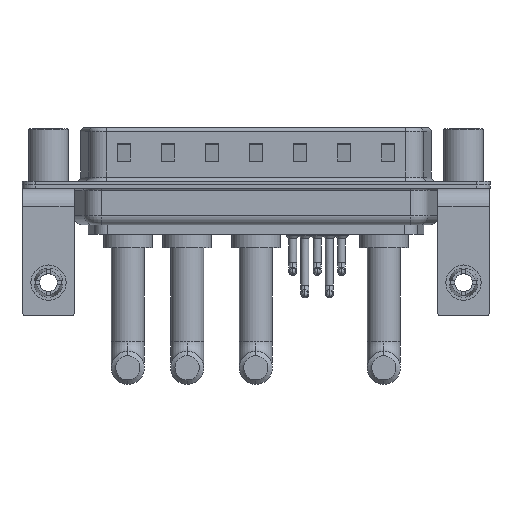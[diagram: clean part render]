
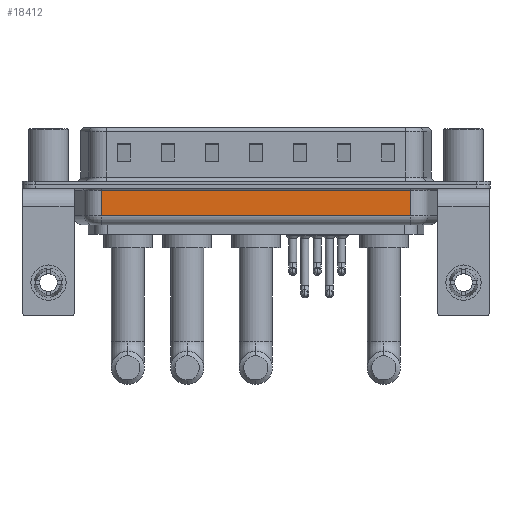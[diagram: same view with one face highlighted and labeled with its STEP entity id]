
A CAD part, front view. The second image highlights one B-rep face of the part: STEP entity #18412.
In plain terms, the highlighted planar face has unit normal (0, -1, 0).
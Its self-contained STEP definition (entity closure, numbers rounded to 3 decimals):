
#325 = ORIENTED_EDGE ( 'NONE', *, *, #12132, .T. ) ;
#992 = DIRECTION ( 'NONE',  ( 0., 0., 1. ) ) ;
#1265 = DIRECTION ( 'NONE',  ( 0., 1., 0. ) ) ;
#1541 = LINE ( 'NONE', #7096, #14160 ) ;
#2260 = CARTESIAN_POINT ( 'NONE',  ( 41.044, -5.35, -3.5 ) ) ;
#2464 = DIRECTION ( 'NONE',  ( 1., 0., 0. ) ) ;
#2958 = LINE ( 'NONE', #11002, #12992 ) ;
#3140 = ORIENTED_EDGE ( 'NONE', *, *, #3337, .F. ) ;
#3337 = EDGE_CURVE ( 'NONE', #5032, #7875, #1541, .T. ) ;
#3889 = LINE ( 'NONE', #17446, #12593 ) ;
#5032 = VERTEX_POINT ( 'NONE', #24955 ) ;
#5621 = ORIENTED_EDGE ( 'NONE', *, *, #23208, .T. ) ;
#5818 = EDGE_LOOP ( 'NONE', ( #3140, #325, #17561, #5621 ) ) ;
#6841 = CARTESIAN_POINT ( 'NONE',  ( 41.044, -5.35, -0.65 ) ) ;
#7096 = CARTESIAN_POINT ( 'NONE',  ( 6.006, -5.35, -4.5 ) ) ;
#7875 = VERTEX_POINT ( 'NONE', #17554 ) ;
#8940 = LINE ( 'NONE', #16942, #12681 ) ;
#11002 = CARTESIAN_POINT ( 'NONE',  ( 41.044, -5.35, -4.5 ) ) ;
#11404 = CARTESIAN_POINT ( 'NONE',  ( 6.006, -5.35, -4.5 ) ) ;
#12132 = EDGE_CURVE ( 'NONE', #5032, #20020, #8940, .T. ) ;
#12593 = VECTOR ( 'NONE', #13364, 1000. ) ;
#12681 = VECTOR ( 'NONE', #2464, 1000. ) ;
#12992 = VECTOR ( 'NONE', #992, 1000. ) ;
#13364 = DIRECTION ( 'NONE',  ( -1., 0., 0. ) ) ;
#14160 = VECTOR ( 'NONE', #23377, 1000. ) ;
#14892 = PLANE ( 'NONE',  #23790 ) ;
#15624 = DIRECTION ( 'NONE',  ( 0., 0., 1. ) ) ;
#16942 = CARTESIAN_POINT ( 'NONE',  ( 6.006, -5.35, -3.5 ) ) ;
#17446 = CARTESIAN_POINT ( 'NONE',  ( 6.006, -5.35, -0.65 ) ) ;
#17554 = CARTESIAN_POINT ( 'NONE',  ( 6.006, -5.35, -0.65 ) ) ;
#17561 = ORIENTED_EDGE ( 'NONE', *, *, #21216, .T. ) ;
#17586 = FACE_OUTER_BOUND ( 'NONE', #5818, .T. ) ;
#18412 = ADVANCED_FACE ( 'NONE', ( #17586 ), #14892, .F. ) ;
#20020 = VERTEX_POINT ( 'NONE', #2260 ) ;
#21216 = EDGE_CURVE ( 'NONE', #20020, #25461, #2958, .T. ) ;
#23208 = EDGE_CURVE ( 'NONE', #25461, #7875, #3889, .T. ) ;
#23377 = DIRECTION ( 'NONE',  ( 0., 0., 1. ) ) ;
#23790 = AXIS2_PLACEMENT_3D ( 'NONE', #11404, #1265, #15624 ) ;
#24955 = CARTESIAN_POINT ( 'NONE',  ( 6.006, -5.35, -3.5 ) ) ;
#25461 = VERTEX_POINT ( 'NONE', #6841 ) ;
